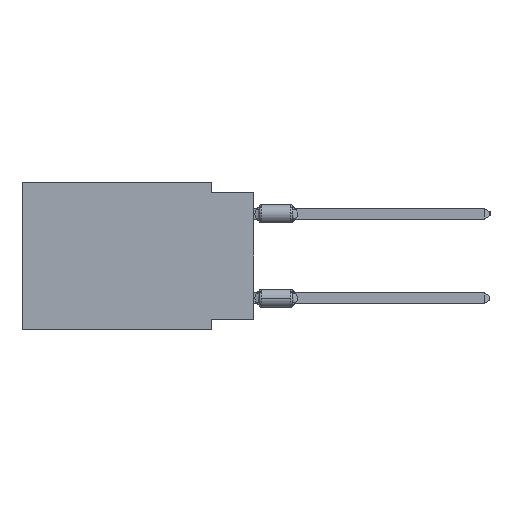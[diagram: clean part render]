
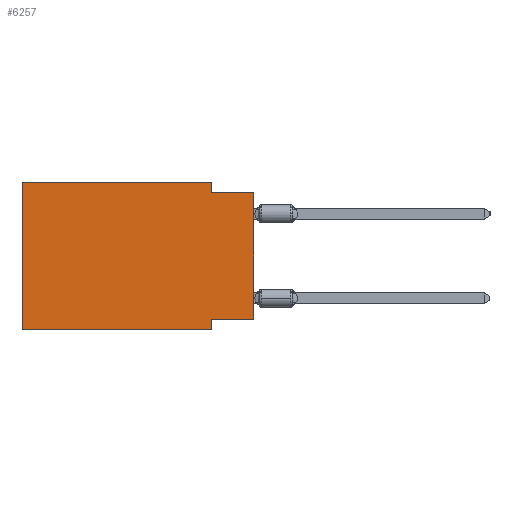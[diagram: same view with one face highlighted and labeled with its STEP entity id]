
A CAD part, left-side view. The second image highlights one B-rep face of the part: STEP entity #6257.
In plain terms, the highlighted planar face has unit normal (-1, 0, 0).
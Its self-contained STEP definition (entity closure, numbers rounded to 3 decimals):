
#129 = DIRECTION ( 'NONE',  ( 0., 1., 0. ) ) ;
#484 = VECTOR ( 'NONE', #7769, 1000. ) ;
#523 = VERTEX_POINT ( 'NONE', #6441 ) ;
#1556 = VECTOR ( 'NONE', #3820, 1000. ) ;
#2118 = EDGE_CURVE ( 'NONE', #14491, #29521, #25842, .T. ) ;
#2163 = LINE ( 'NONE', #21495, #484 ) ;
#3372 = CARTESIAN_POINT ( 'NONE',  ( 0., 0., -8.255 ) ) ;
#3393 = VERTEX_POINT ( 'NONE', #10372 ) ;
#3820 = DIRECTION ( 'NONE',  ( 0., -1., 0. ) ) ;
#3974 = EDGE_CURVE ( 'NONE', #29876, #30386, #10965, .T. ) ;
#6257 = ADVANCED_FACE ( 'NONE', ( #21393 ), #7849, .F. ) ;
#6441 = CARTESIAN_POINT ( 'NONE',  ( 0., 2.54, -8.89 ) ) ;
#6826 = VECTOR ( 'NONE', #20425, 1000. ) ;
#6958 = LINE ( 'NONE', #18447, #11919 ) ;
#7057 = VERTEX_POINT ( 'NONE', #21987 ) ;
#7179 = VECTOR ( 'NONE', #20793, 1000. ) ;
#7769 = DIRECTION ( 'NONE',  ( 0., -1., 0. ) ) ;
#7849 = PLANE ( 'NONE',  #27992 ) ;
#7910 = CARTESIAN_POINT ( 'NONE',  ( 0., 13.97, -8.89 ) ) ;
#8841 = CARTESIAN_POINT ( 'NONE',  ( 0., 0., -8.255 ) ) ;
#8866 = ORIENTED_EDGE ( 'NONE', *, *, #15498, .F. ) ;
#9777 = CARTESIAN_POINT ( 'NONE',  ( 0., 2.54, -8.89 ) ) ;
#10372 = CARTESIAN_POINT ( 'NONE',  ( 0., 2.54, 0. ) ) ;
#10621 = EDGE_CURVE ( 'NONE', #29876, #30634, #31716, .T. ) ;
#10965 = LINE ( 'NONE', #3372, #25967 ) ;
#11919 = VECTOR ( 'NONE', #24055, 1000. ) ;
#12719 = DIRECTION ( 'NONE',  ( 1., 0., 0. ) ) ;
#13372 = ORIENTED_EDGE ( 'NONE', *, *, #2118, .F. ) ;
#14491 = VERTEX_POINT ( 'NONE', #16722 ) ;
#14735 = CARTESIAN_POINT ( 'NONE',  ( 0., 0., 0. ) ) ;
#14808 = CARTESIAN_POINT ( 'NONE',  ( 0., 13.97, 0. ) ) ;
#15498 = EDGE_CURVE ( 'NONE', #30386, #523, #15715, .T. ) ;
#15715 = LINE ( 'NONE', #9777, #7179 ) ;
#16147 = DIRECTION ( 'NONE',  ( 0., 0., -1. ) ) ;
#16722 = CARTESIAN_POINT ( 'NONE',  ( 0., 13.97, -8.89 ) ) ;
#17219 = EDGE_CURVE ( 'NONE', #7057, #30634, #25683, .T. ) ;
#17893 = CARTESIAN_POINT ( 'NONE',  ( 0., 0., -0.635 ) ) ;
#18166 = ORIENTED_EDGE ( 'NONE', *, *, #32478, .F. ) ;
#18447 = CARTESIAN_POINT ( 'NONE',  ( 0., 2.54, 0. ) ) ;
#20425 = DIRECTION ( 'NONE',  ( 0., 0., 1. ) ) ;
#20793 = DIRECTION ( 'NONE',  ( 0., 0., -1. ) ) ;
#21000 = CARTESIAN_POINT ( 'NONE',  ( 0., 2.54, -8.255 ) ) ;
#21029 = CARTESIAN_POINT ( 'NONE',  ( 0., 13.97, 0. ) ) ;
#21393 = FACE_OUTER_BOUND ( 'NONE', #31685, .T. ) ;
#21495 = CARTESIAN_POINT ( 'NONE',  ( 0., 13.97, 0. ) ) ;
#21819 = LINE ( 'NONE', #7910, #35693 ) ;
#21987 = CARTESIAN_POINT ( 'NONE',  ( 0., 2.54, -0.635 ) ) ;
#22775 = ORIENTED_EDGE ( 'NONE', *, *, #17219, .F. ) ;
#22980 = EDGE_CURVE ( 'NONE', #3393, #7057, #6958, .T. ) ;
#23258 = VECTOR ( 'NONE', #29007, 1000. ) ;
#24055 = DIRECTION ( 'NONE',  ( 0., 0., -1. ) ) ;
#25393 = ORIENTED_EDGE ( 'NONE', *, *, #10621, .T. ) ;
#25589 = CARTESIAN_POINT ( 'NONE',  ( 0., 0., -0.635 ) ) ;
#25683 = LINE ( 'NONE', #17893, #1556 ) ;
#25773 = ORIENTED_EDGE ( 'NONE', *, *, #22980, .F. ) ;
#25842 = LINE ( 'NONE', #14808, #6826 ) ;
#25967 = VECTOR ( 'NONE', #129, 1000. ) ;
#26028 = CARTESIAN_POINT ( 'NONE',  ( 0., 13.97, 0. ) ) ;
#27992 = AXIS2_PLACEMENT_3D ( 'NONE', #21029, #12719, #16147 ) ;
#29007 = DIRECTION ( 'NONE',  ( 0., 0., 1. ) ) ;
#29521 = VERTEX_POINT ( 'NONE', #26028 ) ;
#29876 = VERTEX_POINT ( 'NONE', #8841 ) ;
#30386 = VERTEX_POINT ( 'NONE', #21000 ) ;
#30634 = VERTEX_POINT ( 'NONE', #25589 ) ;
#31124 = ORIENTED_EDGE ( 'NONE', *, *, #33040, .T. ) ;
#31685 = EDGE_LOOP ( 'NONE', ( #25393, #22775, #25773, #18166, #13372, #31124, #8866, #33821 ) ) ;
#31716 = LINE ( 'NONE', #14735, #23258 ) ;
#32478 = EDGE_CURVE ( 'NONE', #29521, #3393, #2163, .T. ) ;
#32832 = DIRECTION ( 'NONE',  ( 0., -1., 0. ) ) ;
#33040 = EDGE_CURVE ( 'NONE', #14491, #523, #21819, .T. ) ;
#33821 = ORIENTED_EDGE ( 'NONE', *, *, #3974, .F. ) ;
#35693 = VECTOR ( 'NONE', #32832, 1000. ) ;
